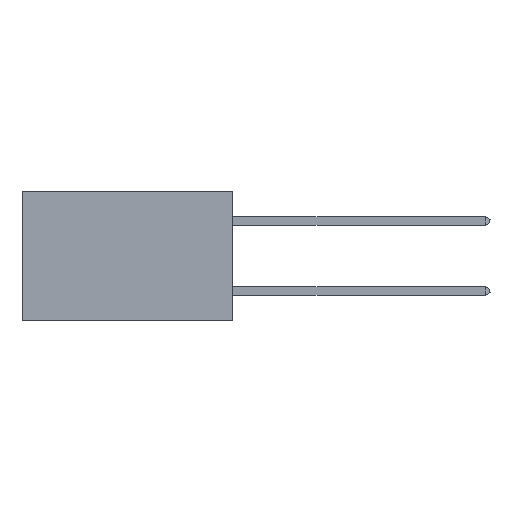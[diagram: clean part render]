
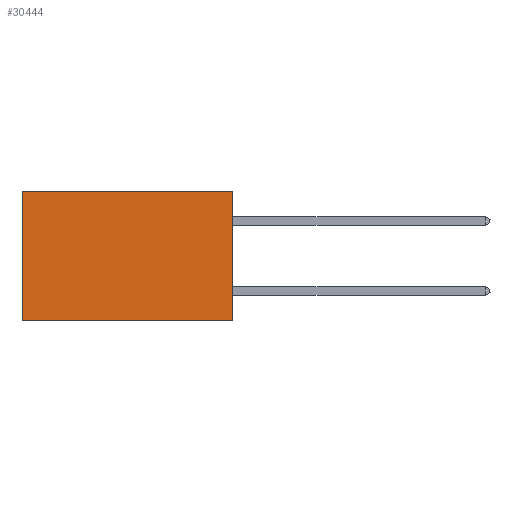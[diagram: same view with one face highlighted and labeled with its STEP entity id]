
A CAD part, left-side view. The second image highlights one B-rep face of the part: STEP entity #30444.
In plain terms, the highlighted planar face has unit normal (-1, 0, 0).
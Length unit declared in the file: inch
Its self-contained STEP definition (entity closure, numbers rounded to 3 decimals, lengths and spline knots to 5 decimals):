
#946 = DIRECTION ( 'NONE',  ( 0., 1., 0. ) ) ;
#1234 = VECTOR ( 'NONE', #19349, 39.37008 ) ;
#1544 = CARTESIAN_POINT ( 'NONE',  ( 0.2875, 0., 0. ) ) ;
#3012 = ORIENTED_EDGE ( 'NONE', *, *, #11427, .F. ) ;
#3813 = CARTESIAN_POINT ( 'NONE',  ( 0.2875, 0.6, -0.37 ) ) ;
#4348 = DIRECTION ( 'NONE',  ( 0., 0., -1. ) ) ;
#4876 = LINE ( 'NONE', #11886, #11302 ) ;
#6641 = CARTESIAN_POINT ( 'NONE',  ( 0.2875, 0.6, 0. ) ) ;
#6653 = EDGE_CURVE ( 'NONE', #13628, #10896, #15643, .T. ) ;
#8540 = LINE ( 'NONE', #16613, #1234 ) ;
#8644 = ORIENTED_EDGE ( 'NONE', *, *, #6653, .T. ) ;
#10896 = VERTEX_POINT ( 'NONE', #3813 ) ;
#11302 = VECTOR ( 'NONE', #946, 39.37008 ) ;
#11427 = EDGE_CURVE ( 'NONE', #27486, #10896, #15028, .T. ) ;
#11886 = CARTESIAN_POINT ( 'NONE',  ( 0.2875, 0., 0. ) ) ;
#12326 = EDGE_LOOP ( 'NONE', ( #8644, #3012, #16342, #34813 ) ) ;
#12653 = DIRECTION ( 'NONE',  ( 0., 0., -1. ) ) ;
#13628 = VERTEX_POINT ( 'NONE', #6641 ) ;
#14160 = VECTOR ( 'NONE', #19318, 39.37008 ) ;
#15028 = LINE ( 'NONE', #19436, #14160 ) ;
#15350 = CARTESIAN_POINT ( 'NONE',  ( 0.2875, 0., -0.37 ) ) ;
#15643 = LINE ( 'NONE', #34331, #22892 ) ;
#16342 = ORIENTED_EDGE ( 'NONE', *, *, #29398, .F. ) ;
#16613 = CARTESIAN_POINT ( 'NONE',  ( 0.2875, 0., 0. ) ) ;
#18193 = VERTEX_POINT ( 'NONE', #34130 ) ;
#19318 = DIRECTION ( 'NONE',  ( 0., 1., 0. ) ) ;
#19349 = DIRECTION ( 'NONE',  ( 0., 0., -1. ) ) ;
#19436 = CARTESIAN_POINT ( 'NONE',  ( 0.2875, 0., -0.37 ) ) ;
#20614 = PLANE ( 'NONE',  #26126 ) ;
#20738 = DIRECTION ( 'NONE',  ( 1., 0., 0. ) ) ;
#22892 = VECTOR ( 'NONE', #12653, 39.37008 ) ;
#26126 = AXIS2_PLACEMENT_3D ( 'NONE', #1544, #20738, #4348 ) ;
#26292 = FACE_OUTER_BOUND ( 'NONE', #12326, .T. ) ;
#26662 = EDGE_CURVE ( 'NONE', #18193, #13628, #4876, .T. ) ;
#27486 = VERTEX_POINT ( 'NONE', #15350 ) ;
#29398 = EDGE_CURVE ( 'NONE', #18193, #27486, #8540, .T. ) ;
#30444 = ADVANCED_FACE ( 'NONE', ( #26292 ), #20614, .F. ) ;
#34130 = CARTESIAN_POINT ( 'NONE',  ( 0.2875, 0., 0. ) ) ;
#34331 = CARTESIAN_POINT ( 'NONE',  ( 0.2875, 0.6, 0. ) ) ;
#34813 = ORIENTED_EDGE ( 'NONE', *, *, #26662, .T. ) ;
